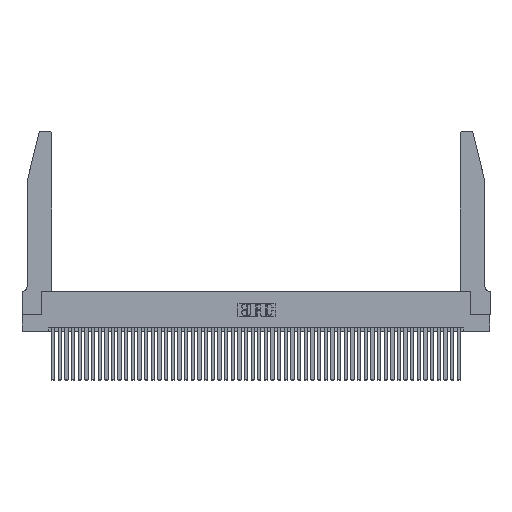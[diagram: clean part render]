
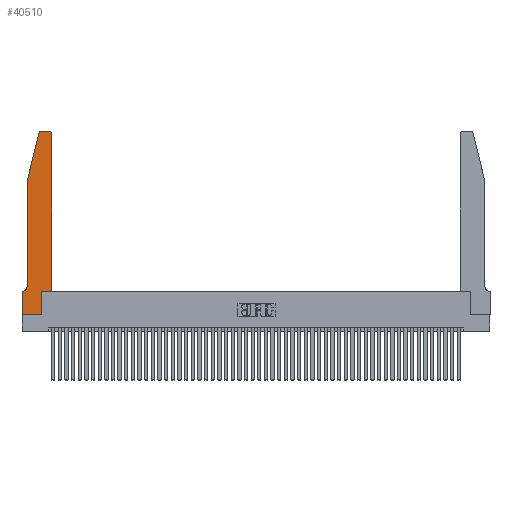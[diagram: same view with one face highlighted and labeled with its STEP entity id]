
A CAD part, top view. The second image highlights one B-rep face of the part: STEP entity #40510.
In plain terms, the highlighted planar face has unit normal (0, 0, 1).
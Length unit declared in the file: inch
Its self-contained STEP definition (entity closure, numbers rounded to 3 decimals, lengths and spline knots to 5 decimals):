
#71 = CARTESIAN_POINT ( 'NONE',  ( 0.25487, 2.72718, 0.37 ) ) ;
#442 = CARTESIAN_POINT ( 'NONE',  ( 0., 0.35, 0.37 ) ) ;
#725 = CARTESIAN_POINT ( 'NONE',  ( 0.0755, 2., 0.37 ) ) ;
#922 = EDGE_CURVE ( 'NONE', #26610, #32968, #20171, .T. ) ;
#1532 = ORIENTED_EDGE ( 'NONE', *, *, #24568, .T. ) ;
#2599 = DIRECTION ( 'NONE',  ( -1., 0., 0. ) ) ;
#3217 = EDGE_CURVE ( 'NONE', #40536, #30143, #41935, .T. ) ;
#3332 = CARTESIAN_POINT ( 'NONE',  ( 0.4205, 2.72, 0.37 ) ) ;
#4313 = VERTEX_POINT ( 'NONE', #36641 ) ;
#4907 = VECTOR ( 'NONE', #45797, 39.37008 ) ;
#5361 = VERTEX_POINT ( 'NONE', #19134 ) ;
#5843 = VERTEX_POINT ( 'NONE', #11098 ) ;
#6288 = PLANE ( 'NONE',  #35556 ) ;
#7048 = ORIENTED_EDGE ( 'NONE', *, *, #20107, .T. ) ;
#7230 = DIRECTION ( 'NONE',  ( 1., 0., 0. ) ) ;
#8125 = ORIENTED_EDGE ( 'NONE', *, *, #35449, .T. ) ;
#8951 = CARTESIAN_POINT ( 'NONE',  ( 0.2865, 0.35, 0.37 ) ) ;
#9190 = CARTESIAN_POINT ( 'NONE',  ( 0.284, 2.72, 0.37 ) ) ;
#9790 = VECTOR ( 'NONE', #40168, 39.37008 ) ;
#10729 = CARTESIAN_POINT ( 'NONE',  ( 0.0055, 0.35, 0.37 ) ) ;
#10961 = ORIENTED_EDGE ( 'NONE', *, *, #45499, .T. ) ;
#11098 = CARTESIAN_POINT ( 'NONE',  ( 0., 0., 0.37 ) ) ;
#11541 = VECTOR ( 'NONE', #19293, 39.37008 ) ;
#12132 = EDGE_CURVE ( 'NONE', #32968, #5361, #37683, .T. ) ;
#13087 = DIRECTION ( 'NONE',  ( 1., 0., 0. ) ) ;
#14094 = DIRECTION ( 'NONE',  ( 1., 0., 0. ) ) ;
#14297 = EDGE_CURVE ( 'NONE', #5361, #40536, #37965, .T. ) ;
#16675 = LINE ( 'NONE', #17541, #27032 ) ;
#17541 = CARTESIAN_POINT ( 'NONE',  ( 0.0755, 2., 0.37 ) ) ;
#17545 = CARTESIAN_POINT ( 'NONE',  ( 0.0055, 0.42, 0.37 ) ) ;
#18024 = CIRCLE ( 'NONE', #19087, 0.03 ) ;
#18026 = CARTESIAN_POINT ( 'NONE',  ( 0.4505, 2.72, 0.37 ) ) ;
#18459 = VECTOR ( 'NONE', #21989, 39.37008 ) ;
#19087 = AXIS2_PLACEMENT_3D ( 'NONE', #9190, #36483, #13087 ) ;
#19134 = CARTESIAN_POINT ( 'NONE',  ( 0.4505, 0.35, 0.37 ) ) ;
#19147 = EDGE_CURVE ( 'NONE', #45397, #25434, #18024, .T. ) ;
#19293 = DIRECTION ( 'NONE',  ( 1., 0., 0. ) ) ;
#19461 = LINE ( 'NONE', #42732, #11541 ) ;
#19698 = LINE ( 'NONE', #49049, #40471 ) ;
#19973 = EDGE_CURVE ( 'NONE', #44562, #4313, #35981, .T. ) ;
#20107 = EDGE_CURVE ( 'NONE', #5843, #26610, #19461, .T. ) ;
#20171 = LINE ( 'NONE', #8951, #9790 ) ;
#20875 = LINE ( 'NONE', #37328, #40421 ) ;
#21279 = DIRECTION ( 'NONE',  ( -0.239, -0.971, 0. ) ) ;
#21455 = DIRECTION ( 'NONE',  ( -1., 0., 0. ) ) ;
#21466 = VERTEX_POINT ( 'NONE', #442 ) ;
#21989 = DIRECTION ( 'NONE',  ( 0., 1., 0. ) ) ;
#22902 = AXIS2_PLACEMENT_3D ( 'NONE', #17545, #44872, #21455 ) ;
#24568 = EDGE_CURVE ( 'NONE', #25434, #44562, #16675, .T. ) ;
#25434 = VERTEX_POINT ( 'NONE', #71 ) ;
#25656 = DIRECTION ( 'NONE',  ( -1., 0., 0. ) ) ;
#25716 = DIRECTION ( 'NONE',  ( 0., 0., 1. ) ) ;
#25952 = ORIENTED_EDGE ( 'NONE', *, *, #36045, .T. ) ;
#26342 = EDGE_CURVE ( 'NONE', #4313, #39839, #46429, .T. ) ;
#26610 = VERTEX_POINT ( 'NONE', #38489 ) ;
#26738 = CARTESIAN_POINT ( 'NONE',  ( 0.2865, 0.35, 0.37 ) ) ;
#27032 = VECTOR ( 'NONE', #21279, 39.37008 ) ;
#30143 = VERTEX_POINT ( 'NONE', #43337 ) ;
#30591 = DIRECTION ( 'NONE',  ( 0., 0., 1. ) ) ;
#32050 = CARTESIAN_POINT ( 'NONE',  ( 0.4505, 0.35, 0.37 ) ) ;
#32730 = FACE_OUTER_BOUND ( 'NONE', #37076, .T. ) ;
#32968 = VERTEX_POINT ( 'NONE', #26738 ) ;
#34386 = ORIENTED_EDGE ( 'NONE', *, *, #922, .T. ) ;
#35449 = EDGE_CURVE ( 'NONE', #39839, #21466, #19698, .T. ) ;
#35556 = AXIS2_PLACEMENT_3D ( 'NONE', #49109, #25716, #14094 ) ;
#35681 = ORIENTED_EDGE ( 'NONE', *, *, #19973, .T. ) ;
#35964 = DIRECTION ( 'NONE',  ( 1., 0., 0. ) ) ;
#35981 = LINE ( 'NONE', #41872, #4907 ) ;
#36045 = EDGE_CURVE ( 'NONE', #30143, #45397, #45924, .T. ) ;
#36483 = DIRECTION ( 'NONE',  ( 0., 0., 1. ) ) ;
#36484 = VECTOR ( 'NONE', #35964, 39.37008 ) ;
#36641 = CARTESIAN_POINT ( 'NONE',  ( 0.0755, 0.42, 0.37 ) ) ;
#37076 = EDGE_LOOP ( 'NONE', ( #25952, #40853, #1532, #35681, #47659, #8125, #10961, #7048, #34386, #46112, #50108, #44557 ) ) ;
#37328 = CARTESIAN_POINT ( 'NONE',  ( 0., 0., 0.37 ) ) ;
#37683 = LINE ( 'NONE', #32050, #36484 ) ;
#37965 = LINE ( 'NONE', #45383, #18459 ) ;
#38489 = CARTESIAN_POINT ( 'NONE',  ( 0.2865, 0., 0.37 ) ) ;
#39839 = VERTEX_POINT ( 'NONE', #10729 ) ;
#40168 = DIRECTION ( 'NONE',  ( 0., 1., 0. ) ) ;
#40421 = VECTOR ( 'NONE', #41285, 39.37008 ) ;
#40471 = VECTOR ( 'NONE', #25656, 39.37008 ) ;
#40510 = ADVANCED_FACE ( 'NONE', ( #32730 ), #6288, .T. ) ;
#40536 = VERTEX_POINT ( 'NONE', #18026 ) ;
#40605 = CARTESIAN_POINT ( 'NONE',  ( 0.284, 2.75, 0.37 ) ) ;
#40853 = ORIENTED_EDGE ( 'NONE', *, *, #19147, .T. ) ;
#41285 = DIRECTION ( 'NONE',  ( 0., -1., 0. ) ) ;
#41289 = CARTESIAN_POINT ( 'NONE',  ( 0.2605, 2.75, 0.37 ) ) ;
#41872 = CARTESIAN_POINT ( 'NONE',  ( 0.0755, 2., 0.37 ) ) ;
#41935 = CIRCLE ( 'NONE', #44018, 0.03 ) ;
#42732 = CARTESIAN_POINT ( 'NONE',  ( 0., 0., 0.37 ) ) ;
#43337 = CARTESIAN_POINT ( 'NONE',  ( 0.4205, 2.75, 0.37 ) ) ;
#44018 = AXIS2_PLACEMENT_3D ( 'NONE', #3332, #30591, #7230 ) ;
#44557 = ORIENTED_EDGE ( 'NONE', *, *, #3217, .T. ) ;
#44562 = VERTEX_POINT ( 'NONE', #725 ) ;
#44717 = VECTOR ( 'NONE', #2599, 39.37008 ) ;
#44872 = DIRECTION ( 'NONE',  ( 0., 0., -1. ) ) ;
#45383 = CARTESIAN_POINT ( 'NONE',  ( 0.4505, 0.35, 0.37 ) ) ;
#45397 = VERTEX_POINT ( 'NONE', #40605 ) ;
#45499 = EDGE_CURVE ( 'NONE', #21466, #5843, #20875, .T. ) ;
#45797 = DIRECTION ( 'NONE',  ( 0., -1., 0. ) ) ;
#45924 = LINE ( 'NONE', #41289, #44717 ) ;
#46112 = ORIENTED_EDGE ( 'NONE', *, *, #12132, .T. ) ;
#46429 = CIRCLE ( 'NONE', #22902, 0.07 ) ;
#47659 = ORIENTED_EDGE ( 'NONE', *, *, #26342, .T. ) ;
#49049 = CARTESIAN_POINT ( 'NONE',  ( 0.0755, 0.35, 0.37 ) ) ;
#49109 = CARTESIAN_POINT ( 'NONE',  ( 0., 0.35, 0.37 ) ) ;
#50108 = ORIENTED_EDGE ( 'NONE', *, *, #14297, .T. ) ;
